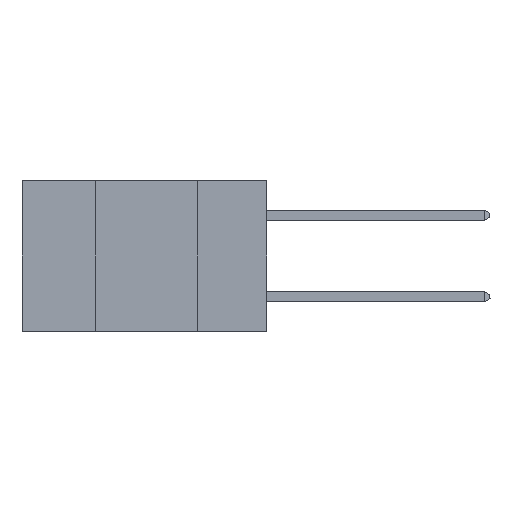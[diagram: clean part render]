
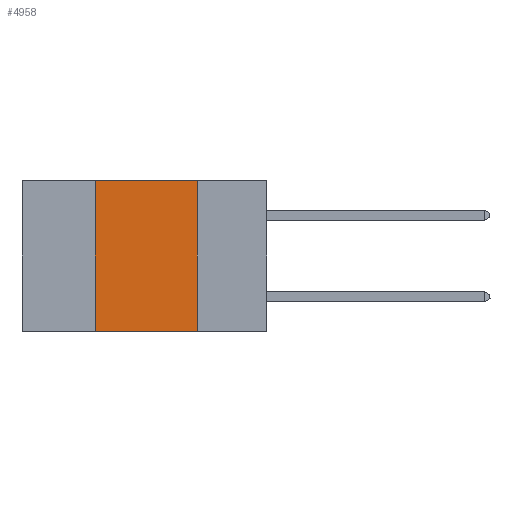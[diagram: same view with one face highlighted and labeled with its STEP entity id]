
A CAD part, left-side view. The second image highlights one B-rep face of the part: STEP entity #4958.
In plain terms, the highlighted planar face has unit normal (-1, 0, 0).
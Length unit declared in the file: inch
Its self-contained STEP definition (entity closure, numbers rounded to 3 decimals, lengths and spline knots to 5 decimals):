
#576 = VERTEX_POINT ( 'NONE', #8452 ) ;
#758 = CARTESIAN_POINT ( 'NONE',  ( 0., 0.42, -0.37 ) ) ;
#1287 = CARTESIAN_POINT ( 'NONE',  ( 0., 0.6, 0. ) ) ;
#1798 = EDGE_CURVE ( 'NONE', #23421, #7947, #20196, .T. ) ;
#2051 = CARTESIAN_POINT ( 'NONE',  ( 0., 0.6, 0. ) ) ;
#3608 = LINE ( 'NONE', #17168, #15404 ) ;
#3943 = CARTESIAN_POINT ( 'NONE',  ( 0., 0.42, 0. ) ) ;
#4079 = LINE ( 'NONE', #1287, #18098 ) ;
#4424 = DIRECTION ( 'NONE',  ( 0., 0., -1. ) ) ;
#4958 = ADVANCED_FACE ( 'NONE', ( #29253 ), #27063, .F. ) ;
#5356 = EDGE_CURVE ( 'NONE', #23421, #27237, #11561, .T. ) ;
#7085 = AXIS2_PLACEMENT_3D ( 'NONE', #2051, #18538, #4424 ) ;
#7116 = VECTOR ( 'NONE', #30472, 39.37008 ) ;
#7402 = EDGE_LOOP ( 'NONE', ( #15466, #13508, #27958, #26900 ) ) ;
#7947 = VERTEX_POINT ( 'NONE', #16412 ) ;
#8452 = CARTESIAN_POINT ( 'NONE',  ( 0., 0.17, 0. ) ) ;
#9237 = DIRECTION ( 'NONE',  ( 0., -1., 0. ) ) ;
#10616 = VECTOR ( 'NONE', #11300, 39.37008 ) ;
#11300 = DIRECTION ( 'NONE',  ( 0., 0., 1. ) ) ;
#11561 = LINE ( 'NONE', #29979, #7116 ) ;
#13508 = ORIENTED_EDGE ( 'NONE', *, *, #27210, .F. ) ;
#15404 = VECTOR ( 'NONE', #21907, 39.37008 ) ;
#15466 = ORIENTED_EDGE ( 'NONE', *, *, #28656, .F. ) ;
#16412 = CARTESIAN_POINT ( 'NONE',  ( 0., 0.42, 0. ) ) ;
#17168 = CARTESIAN_POINT ( 'NONE',  ( 0., 0.17, 0. ) ) ;
#18098 = VECTOR ( 'NONE', #9237, 39.37008 ) ;
#18538 = DIRECTION ( 'NONE',  ( 1., 0., 0. ) ) ;
#20196 = LINE ( 'NONE', #3943, #10616 ) ;
#21907 = DIRECTION ( 'NONE',  ( 0., 0., -1. ) ) ;
#23421 = VERTEX_POINT ( 'NONE', #758 ) ;
#26900 = ORIENTED_EDGE ( 'NONE', *, *, #5356, .T. ) ;
#27063 = PLANE ( 'NONE',  #7085 ) ;
#27210 = EDGE_CURVE ( 'NONE', #7947, #576, #4079, .T. ) ;
#27237 = VERTEX_POINT ( 'NONE', #28505 ) ;
#27958 = ORIENTED_EDGE ( 'NONE', *, *, #1798, .F. ) ;
#28505 = CARTESIAN_POINT ( 'NONE',  ( 0., 0.17, -0.37 ) ) ;
#28656 = EDGE_CURVE ( 'NONE', #576, #27237, #3608, .T. ) ;
#29253 = FACE_OUTER_BOUND ( 'NONE', #7402, .T. ) ;
#29979 = CARTESIAN_POINT ( 'NONE',  ( 0., 0.6, -0.37 ) ) ;
#30472 = DIRECTION ( 'NONE',  ( 0., -1., 0. ) ) ;
